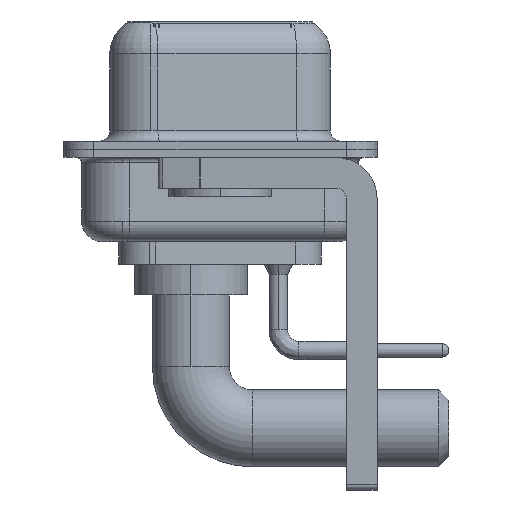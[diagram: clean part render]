
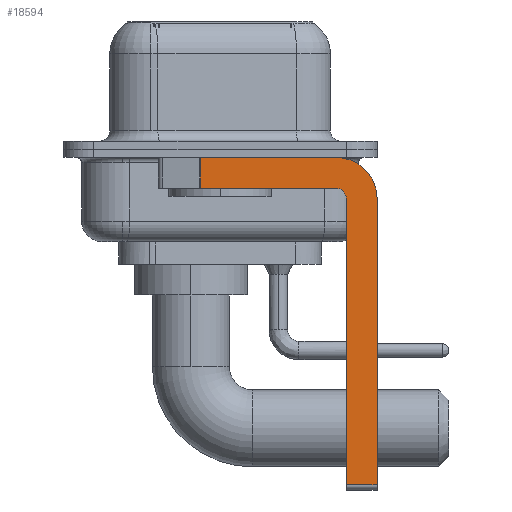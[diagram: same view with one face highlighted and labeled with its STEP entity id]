
A CAD part, left-side view. The second image highlights one B-rep face of the part: STEP entity #18594.
In plain terms, the highlighted planar face has unit normal (-1, 0, 0).
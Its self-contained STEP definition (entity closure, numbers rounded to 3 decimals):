
#381 = CARTESIAN_POINT ( 'NONE',  ( -2.9, -7.65, -2.4 ) ) ;
#609 = ORIENTED_EDGE ( 'NONE', *, *, #14916, .F. ) ;
#691 = VERTEX_POINT ( 'NONE', #16587 ) ;
#921 = ORIENTED_EDGE ( 'NONE', *, *, #8926, .F. ) ;
#1214 = PLANE ( 'NONE',  #10183 ) ;
#1485 = VECTOR ( 'NONE', #9377, 1000. ) ;
#2097 = CIRCLE ( 'NONE', #13780, 2. ) ;
#2386 = CARTESIAN_POINT ( 'NONE',  ( -2.9, -6.15, -16.6 ) ) ;
#2831 = ORIENTED_EDGE ( 'NONE', *, *, #12216, .F. ) ;
#2916 = CARTESIAN_POINT ( 'NONE',  ( -2.9, -6.15, -16.35 ) ) ;
#3049 = VERTEX_POINT ( 'NONE', #10823 ) ;
#3261 = DIRECTION ( 'NONE',  ( 0., -1., 0. ) ) ;
#3649 = CARTESIAN_POINT ( 'NONE',  ( -2.9, 3., -0.4 ) ) ;
#3963 = LINE ( 'NONE', #11043, #8765 ) ;
#3980 = DIRECTION ( 'NONE',  ( 0., -1., 0. ) ) ;
#4427 = AXIS2_PLACEMENT_3D ( 'NONE', #11969, #13517, #10524 ) ;
#4568 = DIRECTION ( 'NONE',  ( 1., 0., 0. ) ) ;
#4879 = VECTOR ( 'NONE', #3261, 1000. ) ;
#4913 = LINE ( 'NONE', #13202, #21269 ) ;
#4958 = DIRECTION ( 'NONE',  ( 0., 0., -1. ) ) ;
#5021 = DIRECTION ( 'NONE',  ( 0., 1., 0. ) ) ;
#5331 = ORIENTED_EDGE ( 'NONE', *, *, #7832, .F. ) ;
#5571 = VERTEX_POINT ( 'NONE', #381 ) ;
#5794 = EDGE_CURVE ( 'NONE', #15482, #8380, #19789, .T. ) ;
#6700 = VERTEX_POINT ( 'NONE', #6827 ) ;
#6827 = CARTESIAN_POINT ( 'NONE',  ( -2.9, -5.65, -0.4 ) ) ;
#7228 = CARTESIAN_POINT ( 'NONE',  ( -2.9, -6.15, -2.4 ) ) ;
#7832 = EDGE_CURVE ( 'NONE', #3049, #6700, #19168, .T. ) ;
#7998 = EDGE_LOOP ( 'NONE', ( #5331, #21718, #921, #609, #2831, #13034, #14004, #12099 ) ) ;
#8124 = EDGE_CURVE ( 'NONE', #6700, #5571, #2097, .T. ) ;
#8158 = CARTESIAN_POINT ( 'NONE',  ( -2.9, -5.65, -2.4 ) ) ;
#8255 = LINE ( 'NONE', #11593, #19793 ) ;
#8380 = VERTEX_POINT ( 'NONE', #21041 ) ;
#8765 = VECTOR ( 'NONE', #14167, 1000. ) ;
#8926 = EDGE_CURVE ( 'NONE', #14444, #691, #4913, .T. ) ;
#9377 = DIRECTION ( 'NONE',  ( 0., 0., 1. ) ) ;
#9942 = DIRECTION ( 'NONE',  ( 0., 0., -1. ) ) ;
#10055 = DIRECTION ( 'NONE',  ( 1., 0., 0. ) ) ;
#10183 = AXIS2_PLACEMENT_3D ( 'NONE', #19536, #4568, #14541 ) ;
#10227 = CARTESIAN_POINT ( 'NONE',  ( -2.9, -5.65, -1.9 ) ) ;
#10524 = DIRECTION ( 'NONE',  ( 0., 0., 1. ) ) ;
#10823 = CARTESIAN_POINT ( 'NONE',  ( -2.9, 0.978, -0.4 ) ) ;
#11043 = CARTESIAN_POINT ( 'NONE',  ( -2.9, 0.978, -1.9 ) ) ;
#11321 = FACE_OUTER_BOUND ( 'NONE', #7998, .T. ) ;
#11593 = CARTESIAN_POINT ( 'NONE',  ( -2.9, -7.65, -2.4 ) ) ;
#11969 = CARTESIAN_POINT ( 'NONE',  ( -2.9, -5.65, -2.4 ) ) ;
#12099 = ORIENTED_EDGE ( 'NONE', *, *, #8124, .F. ) ;
#12216 = EDGE_CURVE ( 'NONE', #15482, #19739, #14272, .T. ) ;
#13034 = ORIENTED_EDGE ( 'NONE', *, *, #5794, .T. ) ;
#13202 = CARTESIAN_POINT ( 'NONE',  ( -2.9, -5.65, -1.9 ) ) ;
#13517 = DIRECTION ( 'NONE',  ( -1., 0., 0. ) ) ;
#13780 = AXIS2_PLACEMENT_3D ( 'NONE', #8158, #10055, #9942 ) ;
#14004 = ORIENTED_EDGE ( 'NONE', *, *, #20981, .F. ) ;
#14167 = DIRECTION ( 'NONE',  ( 0., 0., -1. ) ) ;
#14272 = LINE ( 'NONE', #2386, #1485 ) ;
#14444 = VERTEX_POINT ( 'NONE', #10227 ) ;
#14541 = DIRECTION ( 'NONE',  ( 0., 0., -1. ) ) ;
#14916 = EDGE_CURVE ( 'NONE', #19739, #14444, #16108, .T. ) ;
#15482 = VERTEX_POINT ( 'NONE', #2916 ) ;
#16108 = CIRCLE ( 'NONE', #4427, 0.5 ) ;
#16452 = CARTESIAN_POINT ( 'NONE',  ( -2.9, -5.65, -16.35 ) ) ;
#16587 = CARTESIAN_POINT ( 'NONE',  ( -2.9, 0.978, -1.9 ) ) ;
#18594 = ADVANCED_FACE ( 'NONE', ( #11321 ), #1214, .F. ) ;
#19156 = EDGE_CURVE ( 'NONE', #3049, #691, #3963, .T. ) ;
#19168 = LINE ( 'NONE', #3649, #19441 ) ;
#19441 = VECTOR ( 'NONE', #3980, 1000. ) ;
#19536 = CARTESIAN_POINT ( 'NONE',  ( -2.9, -5.65, -2.4 ) ) ;
#19739 = VERTEX_POINT ( 'NONE', #7228 ) ;
#19789 = LINE ( 'NONE', #16452, #4879 ) ;
#19793 = VECTOR ( 'NONE', #4958, 1000. ) ;
#20981 = EDGE_CURVE ( 'NONE', #5571, #8380, #8255, .T. ) ;
#21041 = CARTESIAN_POINT ( 'NONE',  ( -2.9, -7.65, -16.35 ) ) ;
#21269 = VECTOR ( 'NONE', #5021, 1000. ) ;
#21718 = ORIENTED_EDGE ( 'NONE', *, *, #19156, .T. ) ;
